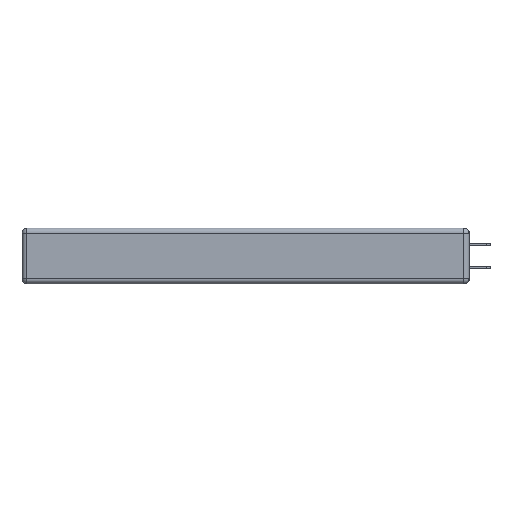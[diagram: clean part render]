
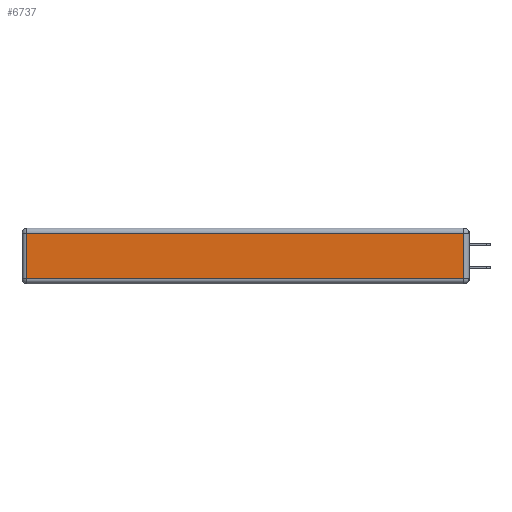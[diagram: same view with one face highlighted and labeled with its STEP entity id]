
A CAD part, left-side view. The second image highlights one B-rep face of the part: STEP entity #6737.
In plain terms, the highlighted planar face has unit normal (-1, 0, 0).
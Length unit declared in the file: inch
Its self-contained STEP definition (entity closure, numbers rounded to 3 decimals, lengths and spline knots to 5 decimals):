
#6 = DIRECTION ( 'NONE',  ( 0., 1., 0. ) ) ;
#79 = LINE ( 'NONE', #9226, #987 ) ;
#987 = VECTOR ( 'NONE', #5035, 39.37008 ) ;
#3171 = ORIENTED_EDGE ( 'NONE', *, *, #11403, .T. ) ;
#3855 = VERTEX_POINT ( 'NONE', #9392 ) ;
#3859 = CARTESIAN_POINT ( 'NONE',  ( 0., 2.75, -0.03 ) ) ;
#3926 = VECTOR ( 'NONE', #13409, 39.37008 ) ;
#4942 = LINE ( 'NONE', #12308, #15919 ) ;
#5035 = DIRECTION ( 'NONE',  ( 0., 0., 1. ) ) ;
#5215 = CARTESIAN_POINT ( 'NONE',  ( 0., 0.03, -0.03 ) ) ;
#6732 = DIRECTION ( 'NONE',  ( 0., -1., 0. ) ) ;
#6737 = ADVANCED_FACE ( 'NONE', ( #17105 ), #11123, .T. ) ;
#6905 = ORIENTED_EDGE ( 'NONE', *, *, #15923, .T. ) ;
#7809 = CARTESIAN_POINT ( 'NONE',  ( 0., 2.72, -0.343 ) ) ;
#8230 = DIRECTION ( 'NONE',  ( -1., 0., 0. ) ) ;
#8295 = DIRECTION ( 'NONE',  ( 0., 0., 1. ) ) ;
#9226 = CARTESIAN_POINT ( 'NONE',  ( 0., 0.03, -0.343 ) ) ;
#9392 = CARTESIAN_POINT ( 'NONE',  ( 0., 0.03, -0.313 ) ) ;
#9585 = CARTESIAN_POINT ( 'NONE',  ( 0., 2.72, -0.313 ) ) ;
#9738 = ORIENTED_EDGE ( 'NONE', *, *, #10549, .T. ) ;
#10549 = EDGE_CURVE ( 'NONE', #3855, #15461, #79, .T. ) ;
#10757 = VERTEX_POINT ( 'NONE', #9585 ) ;
#10889 = VECTOR ( 'NONE', #6, 39.37008 ) ;
#11123 = PLANE ( 'NONE',  #15680 ) ;
#11403 = EDGE_CURVE ( 'NONE', #15461, #15398, #15750, .T. ) ;
#11833 = CARTESIAN_POINT ( 'NONE',  ( 0., 2.72, -0.03 ) ) ;
#12308 = CARTESIAN_POINT ( 'NONE',  ( 0., 0., -0.313 ) ) ;
#13409 = DIRECTION ( 'NONE',  ( 0., 0., -1. ) ) ;
#14233 = LINE ( 'NONE', #7809, #3926 ) ;
#15398 = VERTEX_POINT ( 'NONE', #11833 ) ;
#15429 = CARTESIAN_POINT ( 'NONE',  ( 0., 0., -0.343 ) ) ;
#15461 = VERTEX_POINT ( 'NONE', #5215 ) ;
#15680 = AXIS2_PLACEMENT_3D ( 'NONE', #15429, #8230, #8295 ) ;
#15750 = LINE ( 'NONE', #3859, #10889 ) ;
#15919 = VECTOR ( 'NONE', #6732, 39.37008 ) ;
#15923 = EDGE_CURVE ( 'NONE', #15398, #10757, #14233, .T. ) ;
#17105 = FACE_OUTER_BOUND ( 'NONE', #17881, .T. ) ;
#17218 = ORIENTED_EDGE ( 'NONE', *, *, #18335, .T. ) ;
#17881 = EDGE_LOOP ( 'NONE', ( #17218, #9738, #3171, #6905 ) ) ;
#18335 = EDGE_CURVE ( 'NONE', #10757, #3855, #4942, .T. ) ;
